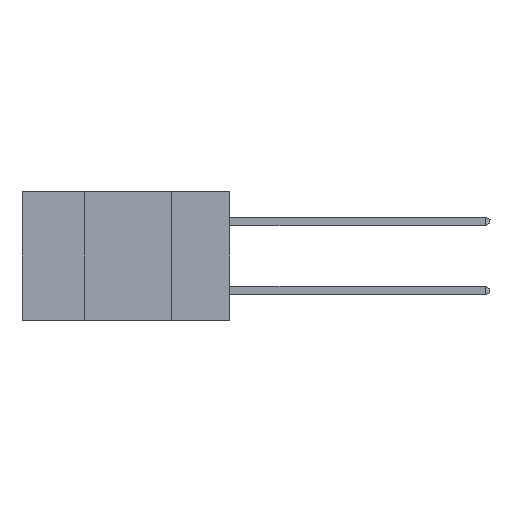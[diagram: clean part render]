
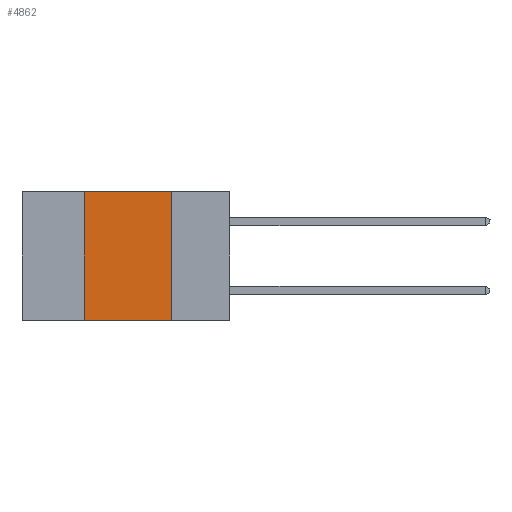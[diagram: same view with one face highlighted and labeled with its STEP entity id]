
A CAD part, left-side view. The second image highlights one B-rep face of the part: STEP entity #4862.
In plain terms, the highlighted planar face has unit normal (-1, 0, 0).
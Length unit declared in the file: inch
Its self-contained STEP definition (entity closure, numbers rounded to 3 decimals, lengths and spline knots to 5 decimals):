
#290 = LINE ( 'NONE', #3572, #16854 ) ;
#1473 = CARTESIAN_POINT ( 'NONE',  ( 0., 0.17, -0.37 ) ) ;
#1765 = FACE_OUTER_BOUND ( 'NONE', #3914, .T. ) ;
#2162 = DIRECTION ( 'NONE',  ( 0., -1., 0. ) ) ;
#2208 = VERTEX_POINT ( 'NONE', #8618 ) ;
#3171 = ORIENTED_EDGE ( 'NONE', *, *, #6179, .F. ) ;
#3179 = DIRECTION ( 'NONE',  ( 0., -1., 0. ) ) ;
#3413 = AXIS2_PLACEMENT_3D ( 'NONE', #10722, #9525, #8843 ) ;
#3455 = DIRECTION ( 'NONE',  ( 0., 0., -1. ) ) ;
#3572 = CARTESIAN_POINT ( 'NONE',  ( 0., 0.17, -0.37 ) ) ;
#3914 = EDGE_LOOP ( 'NONE', ( #8676, #3171, #17448, #13242 ) ) ;
#4465 = VECTOR ( 'NONE', #7022, 39.37008 ) ;
#4862 = ADVANCED_FACE ( 'NONE', ( #1765 ), #14766, .F. ) ;
#6179 = EDGE_CURVE ( 'NONE', #11836, #2208, #11024, .T. ) ;
#7022 = DIRECTION ( 'NONE',  ( 0., 0., 1. ) ) ;
#7611 = CARTESIAN_POINT ( 'NONE',  ( 0., 0.42, -0.37 ) ) ;
#8618 = CARTESIAN_POINT ( 'NONE',  ( 0., 0.17, 0. ) ) ;
#8676 = ORIENTED_EDGE ( 'NONE', *, *, #13841, .F. ) ;
#8762 = LINE ( 'NONE', #21371, #4465 ) ;
#8843 = DIRECTION ( 'NONE',  ( 0., 0., -1. ) ) ;
#9525 = DIRECTION ( 'NONE',  ( 1., 0., 0. ) ) ;
#10722 = CARTESIAN_POINT ( 'NONE',  ( 0., 0.6, 0. ) ) ;
#10973 = EDGE_CURVE ( 'NONE', #13043, #13692, #19131, .T. ) ;
#11024 = LINE ( 'NONE', #18120, #11639 ) ;
#11639 = VECTOR ( 'NONE', #2162, 39.37008 ) ;
#11836 = VERTEX_POINT ( 'NONE', #14421 ) ;
#13043 = VERTEX_POINT ( 'NONE', #7611 ) ;
#13242 = ORIENTED_EDGE ( 'NONE', *, *, #10973, .T. ) ;
#13692 = VERTEX_POINT ( 'NONE', #1473 ) ;
#13760 = CARTESIAN_POINT ( 'NONE',  ( 0., 0.6, -0.37 ) ) ;
#13841 = EDGE_CURVE ( 'NONE', #2208, #13692, #290, .T. ) ;
#14421 = CARTESIAN_POINT ( 'NONE',  ( 0., 0.42, 0. ) ) ;
#14766 = PLANE ( 'NONE',  #3413 ) ;
#15303 = VECTOR ( 'NONE', #3179, 39.37008 ) ;
#16854 = VECTOR ( 'NONE', #3455, 39.37008 ) ;
#17448 = ORIENTED_EDGE ( 'NONE', *, *, #19308, .F. ) ;
#18120 = CARTESIAN_POINT ( 'NONE',  ( 0., 0.6, 0. ) ) ;
#19131 = LINE ( 'NONE', #13760, #15303 ) ;
#19308 = EDGE_CURVE ( 'NONE', #13043, #11836, #8762, .T. ) ;
#21371 = CARTESIAN_POINT ( 'NONE',  ( 0., 0.42, -0.37 ) ) ;
